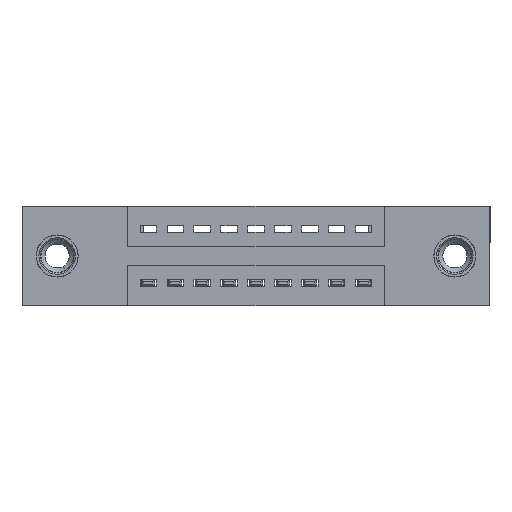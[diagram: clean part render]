
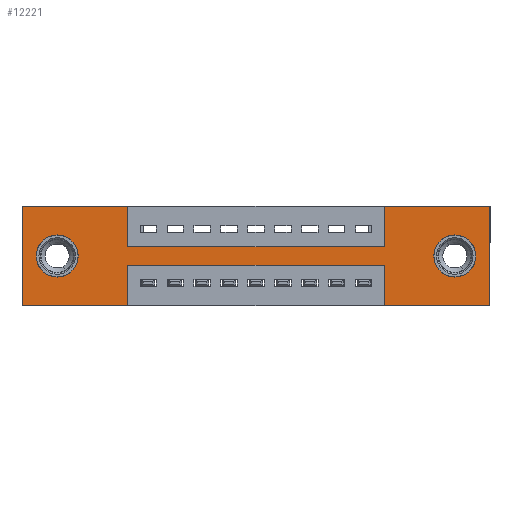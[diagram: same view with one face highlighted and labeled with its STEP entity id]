
A CAD part, front view. The second image highlights one B-rep face of the part: STEP entity #12221.
In plain terms, the highlighted planar face has unit normal (0, -1, 0).
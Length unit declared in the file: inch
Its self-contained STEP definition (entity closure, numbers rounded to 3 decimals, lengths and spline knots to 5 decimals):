
#45 = ORIENTED_EDGE ( 'NONE', *, *, #14666, .F. ) ;
#111 = ORIENTED_EDGE ( 'NONE', *, *, #5245, .F. ) ;
#118 = VERTEX_POINT ( 'NONE', #5059 ) ;
#217 = VECTOR ( 'NONE', #11355, 39.37008 ) ;
#269 = EDGE_CURVE ( 'NONE', #9128, #933, #7332, .T. ) ;
#306 = AXIS2_PLACEMENT_3D ( 'NONE', #4884, #4782, #9347 ) ;
#338 = EDGE_CURVE ( 'NONE', #4870, #15518, #11704, .T. ) ;
#825 = DIRECTION ( 'NONE',  ( 0., 1., 0. ) ) ;
#925 = CARTESIAN_POINT ( 'NONE',  ( 0.13, 0., -0.185 ) ) ;
#933 = VERTEX_POINT ( 'NONE', #5445 ) ;
#942 = ORIENTED_EDGE ( 'NONE', *, *, #8628, .T. ) ;
#1063 = EDGE_CURVE ( 'NONE', #15131, #7904, #8072, .T. ) ;
#1641 = ORIENTED_EDGE ( 'NONE', *, *, #12492, .F. ) ;
#1704 = CARTESIAN_POINT ( 'NONE',  ( 0.3925, 0., -0.22 ) ) ;
#1917 = LINE ( 'NONE', #3874, #8553 ) ;
#1960 = DIRECTION ( 'NONE',  ( 0., 1., 0. ) ) ;
#2021 = DIRECTION ( 'NONE',  ( 0., 0., 1. ) ) ;
#2073 = CARTESIAN_POINT ( 'NONE',  ( 1.605, 0., -0.185 ) ) ;
#2143 = FACE_BOUND ( 'NONE', #11558, .T. ) ;
#2261 = VECTOR ( 'NONE', #4734, 39.37008 ) ;
#2611 = EDGE_CURVE ( 'NONE', #3194, #9128, #13757, .T. ) ;
#3072 = EDGE_CURVE ( 'NONE', #12019, #6812, #7316, .T. ) ;
#3107 = FACE_OUTER_BOUND ( 'NONE', #11637, .T. ) ;
#3136 = ORIENTED_EDGE ( 'NONE', *, *, #6891, .F. ) ;
#3194 = VERTEX_POINT ( 'NONE', #14440 ) ;
#3594 = LINE ( 'NONE', #8298, #2261 ) ;
#3597 = CARTESIAN_POINT ( 'NONE',  ( 0.3925, 0., -0.15 ) ) ;
#3676 = DIRECTION ( 'NONE',  ( 0., 0., 1. ) ) ;
#3874 = CARTESIAN_POINT ( 'NONE',  ( 0.3925, 0., 0. ) ) ;
#3880 = CARTESIAN_POINT ( 'NONE',  ( 1.3425, 0., 0. ) ) ;
#3914 = VECTOR ( 'NONE', #10118, 39.37008 ) ;
#4007 = CARTESIAN_POINT ( 'NONE',  ( 0., 0., -0.37 ) ) ;
#4113 = LINE ( 'NONE', #11731, #9998 ) ;
#4434 = ORIENTED_EDGE ( 'NONE', *, *, #3072, .T. ) ;
#4534 = ORIENTED_EDGE ( 'NONE', *, *, #2611, .F. ) ;
#4734 = DIRECTION ( 'NONE',  ( 0., 0., 1. ) ) ;
#4782 = DIRECTION ( 'NONE',  ( 0., 1., 0. ) ) ;
#4831 = DIRECTION ( 'NONE',  ( 0., 0., 1. ) ) ;
#4870 = VERTEX_POINT ( 'NONE', #9847 ) ;
#4884 = CARTESIAN_POINT ( 'NONE',  ( 0.13, 0., -0.185 ) ) ;
#5059 = CARTESIAN_POINT ( 'NONE',  ( 0.3925, 0., 0. ) ) ;
#5245 = EDGE_CURVE ( 'NONE', #6628, #8516, #4113, .T. ) ;
#5378 = EDGE_LOOP ( 'NONE', ( #4434, #9911 ) ) ;
#5415 = CARTESIAN_POINT ( 'NONE',  ( 0., 0., -0.37 ) ) ;
#5445 = CARTESIAN_POINT ( 'NONE',  ( 0.3925, 0., -0.37 ) ) ;
#5629 = ORIENTED_EDGE ( 'NONE', *, *, #9000, .F. ) ;
#5645 = CARTESIAN_POINT ( 'NONE',  ( 0., 0., -0.37 ) ) ;
#5750 = DIRECTION ( 'NONE',  ( 1., 0., 0. ) ) ;
#5794 = CARTESIAN_POINT ( 'NONE',  ( 0., 0., 0. ) ) ;
#5815 = CARTESIAN_POINT ( 'NONE',  ( 1.3425, 0., -0.15 ) ) ;
#5850 = CARTESIAN_POINT ( 'NONE',  ( 1.735, 0., 0. ) ) ;
#5877 = EDGE_CURVE ( 'NONE', #11410, #15232, #12447, .T. ) ;
#6221 = CARTESIAN_POINT ( 'NONE',  ( 1.735, 0., 0. ) ) ;
#6445 = CARTESIAN_POINT ( 'NONE',  ( 0.3925, 0., -0.37 ) ) ;
#6499 = AXIS2_PLACEMENT_3D ( 'NONE', #2073, #825, #12939 ) ;
#6513 = VECTOR ( 'NONE', #8056, 39.37008 ) ;
#6628 = VERTEX_POINT ( 'NONE', #3880 ) ;
#6812 = VERTEX_POINT ( 'NONE', #14485 ) ;
#6813 = PLANE ( 'NONE',  #12146 ) ;
#6891 = EDGE_CURVE ( 'NONE', #15518, #3194, #14534, .T. ) ;
#7039 = VECTOR ( 'NONE', #3676, 39.37008 ) ;
#7196 = DIRECTION ( 'NONE',  ( 0., 0., -1. ) ) ;
#7316 = CIRCLE ( 'NONE', #8881, 0.078 ) ;
#7332 = LINE ( 'NONE', #6445, #15526 ) ;
#7450 = DIRECTION ( 'NONE',  ( 1., 0., 0. ) ) ;
#7662 = CARTESIAN_POINT ( 'NONE',  ( 1.605, 0., -0.107 ) ) ;
#7666 = VECTOR ( 'NONE', #7196, 39.37008 ) ;
#7904 = VERTEX_POINT ( 'NONE', #5815 ) ;
#7982 = DIRECTION ( 'NONE',  ( 0., 0., -1. ) ) ;
#8056 = DIRECTION ( 'NONE',  ( 1., 0., 0. ) ) ;
#8072 = LINE ( 'NONE', #13534, #11686 ) ;
#8250 = ORIENTED_EDGE ( 'NONE', *, *, #12606, .F. ) ;
#8298 = CARTESIAN_POINT ( 'NONE',  ( 1.3425, 0., 0. ) ) ;
#8404 = LINE ( 'NONE', #5850, #7666 ) ;
#8436 = CARTESIAN_POINT ( 'NONE',  ( 1.3425, 0., -0.37 ) ) ;
#8516 = VERTEX_POINT ( 'NONE', #6221 ) ;
#8553 = VECTOR ( 'NONE', #9867, 39.37008 ) ;
#8581 = CARTESIAN_POINT ( 'NONE',  ( 0., 0., 0. ) ) ;
#8614 = LINE ( 'NONE', #10085, #217 ) ;
#8628 = EDGE_CURVE ( 'NONE', #15232, #11410, #8732, .T. ) ;
#8699 = ORIENTED_EDGE ( 'NONE', *, *, #13551, .F. ) ;
#8714 = CARTESIAN_POINT ( 'NONE',  ( 0.13, 0., -0.107 ) ) ;
#8732 = CIRCLE ( 'NONE', #6499, 0.078 ) ;
#8881 = AXIS2_PLACEMENT_3D ( 'NONE', #925, #10693, #2021 ) ;
#9000 = EDGE_CURVE ( 'NONE', #7904, #6628, #3594, .T. ) ;
#9128 = VERTEX_POINT ( 'NONE', #11361 ) ;
#9347 = DIRECTION ( 'NONE',  ( 0., 0., 1. ) ) ;
#9712 = CARTESIAN_POINT ( 'NONE',  ( 1.605, 0., -0.263 ) ) ;
#9847 = CARTESIAN_POINT ( 'NONE',  ( 1.735, 0., -0.37 ) ) ;
#9867 = DIRECTION ( 'NONE',  ( 0., 0., -1. ) ) ;
#9911 = ORIENTED_EDGE ( 'NONE', *, *, #12916, .T. ) ;
#9998 = VECTOR ( 'NONE', #5750, 39.37008 ) ;
#10085 = CARTESIAN_POINT ( 'NONE',  ( 0., 0., -0.37 ) ) ;
#10118 = DIRECTION ( 'NONE',  ( -1., 0., 0. ) ) ;
#10137 = VECTOR ( 'NONE', #4831, 39.37008 ) ;
#10693 = DIRECTION ( 'NONE',  ( 0., 1., 0. ) ) ;
#11247 = ORIENTED_EDGE ( 'NONE', *, *, #1063, .F. ) ;
#11354 = VERTEX_POINT ( 'NONE', #13673 ) ;
#11355 = DIRECTION ( 'NONE',  ( -1., 0., 0. ) ) ;
#11361 = CARTESIAN_POINT ( 'NONE',  ( 0.3925, 0., -0.22 ) ) ;
#11410 = VERTEX_POINT ( 'NONE', #7662 ) ;
#11505 = DIRECTION ( 'NONE',  ( -1., 0., 0. ) ) ;
#11558 = EDGE_LOOP ( 'NONE', ( #13685, #942 ) ) ;
#11595 = DIRECTION ( 'NONE',  ( 0., 0., -1. ) ) ;
#11637 = EDGE_LOOP ( 'NONE', ( #14683, #4534, #3136, #13594, #8250, #111, #5629, #11247, #8699, #1641, #45, #14971 ) ) ;
#11673 = FACE_BOUND ( 'NONE', #5378, .T. ) ;
#11686 = VECTOR ( 'NONE', #7450, 39.37008 ) ;
#11704 = LINE ( 'NONE', #4007, #3914 ) ;
#11731 = CARTESIAN_POINT ( 'NONE',  ( 0., 0., 0. ) ) ;
#11807 = EDGE_CURVE ( 'NONE', #933, #12357, #8614, .T. ) ;
#12019 = VERTEX_POINT ( 'NONE', #8714 ) ;
#12036 = LINE ( 'NONE', #5794, #6513 ) ;
#12146 = AXIS2_PLACEMENT_3D ( 'NONE', #5415, #14014, #11595 ) ;
#12221 = ADVANCED_FACE ( 'NONE', ( #2143, #11673, #3107 ), #6813, .T. ) ;
#12357 = VERTEX_POINT ( 'NONE', #5645 ) ;
#12447 = CIRCLE ( 'NONE', #13318, 0.078 ) ;
#12492 = EDGE_CURVE ( 'NONE', #11354, #118, #12036, .T. ) ;
#12606 = EDGE_CURVE ( 'NONE', #8516, #4870, #8404, .T. ) ;
#12916 = EDGE_CURVE ( 'NONE', #6812, #12019, #13960, .T. ) ;
#12939 = DIRECTION ( 'NONE',  ( 0., 0., -1. ) ) ;
#12977 = CARTESIAN_POINT ( 'NONE',  ( 1.605, 0., -0.185 ) ) ;
#13318 = AXIS2_PLACEMENT_3D ( 'NONE', #12977, #1960, #7982 ) ;
#13534 = CARTESIAN_POINT ( 'NONE',  ( 0.3925, 0., -0.15 ) ) ;
#13551 = EDGE_CURVE ( 'NONE', #118, #15131, #1917, .T. ) ;
#13594 = ORIENTED_EDGE ( 'NONE', *, *, #338, .F. ) ;
#13673 = CARTESIAN_POINT ( 'NONE',  ( 0., 0., 0. ) ) ;
#13685 = ORIENTED_EDGE ( 'NONE', *, *, #5877, .T. ) ;
#13757 = LINE ( 'NONE', #1704, #15284 ) ;
#13960 = CIRCLE ( 'NONE', #306, 0.078 ) ;
#14014 = DIRECTION ( 'NONE',  ( 0., -1., 0. ) ) ;
#14440 = CARTESIAN_POINT ( 'NONE',  ( 1.3425, 0., -0.22 ) ) ;
#14485 = CARTESIAN_POINT ( 'NONE',  ( 0.13, 0., -0.263 ) ) ;
#14534 = LINE ( 'NONE', #8436, #10137 ) ;
#14641 = LINE ( 'NONE', #8581, #7039 ) ;
#14666 = EDGE_CURVE ( 'NONE', #12357, #11354, #14641, .T. ) ;
#14683 = ORIENTED_EDGE ( 'NONE', *, *, #269, .F. ) ;
#14971 = ORIENTED_EDGE ( 'NONE', *, *, #11807, .F. ) ;
#15058 = DIRECTION ( 'NONE',  ( 0., 0., -1. ) ) ;
#15131 = VERTEX_POINT ( 'NONE', #3597 ) ;
#15232 = VERTEX_POINT ( 'NONE', #9712 ) ;
#15284 = VECTOR ( 'NONE', #11505, 39.37008 ) ;
#15300 = CARTESIAN_POINT ( 'NONE',  ( 1.3425, 0., -0.37 ) ) ;
#15518 = VERTEX_POINT ( 'NONE', #15300 ) ;
#15526 = VECTOR ( 'NONE', #15058, 39.37008 ) ;
